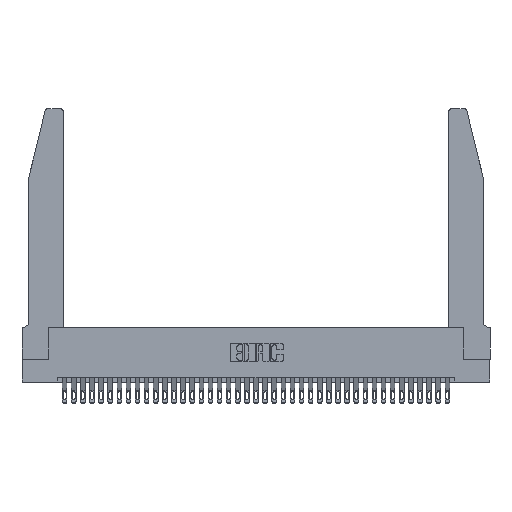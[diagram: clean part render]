
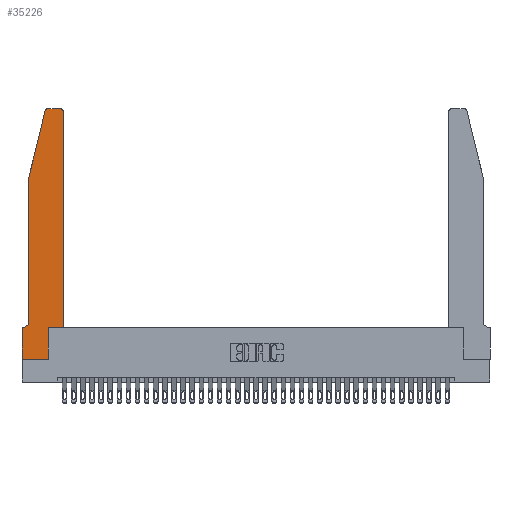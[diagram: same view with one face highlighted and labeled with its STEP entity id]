
A CAD part, top view. The second image highlights one B-rep face of the part: STEP entity #35226.
In plain terms, the highlighted planar face has unit normal (0, 0, 1).
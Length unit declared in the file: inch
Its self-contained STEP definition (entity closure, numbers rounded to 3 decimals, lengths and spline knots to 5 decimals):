
#294 = EDGE_CURVE ( 'NONE', #10274, #26680, #36121, .T. ) ;
#862 = LINE ( 'NONE', #12136, #24023 ) ;
#1189 = LINE ( 'NONE', #4709, #31174 ) ;
#1257 = VERTEX_POINT ( 'NONE', #12791 ) ;
#2645 = EDGE_CURVE ( 'NONE', #26680, #19463, #24543, .T. ) ;
#2766 = ORIENTED_EDGE ( 'NONE', *, *, #25199, .T. ) ;
#3398 = EDGE_CURVE ( 'NONE', #1257, #34797, #37772, .T. ) ;
#3611 = CARTESIAN_POINT ( 'NONE',  ( 0.4505, 0.35, 0.37 ) ) ;
#3882 = DIRECTION ( 'NONE',  ( 0., 1., 0. ) ) ;
#4219 = DIRECTION ( 'NONE',  ( 0., 0., -1. ) ) ;
#4265 = CARTESIAN_POINT ( 'NONE',  ( 0.2865, 0.35, 0.37 ) ) ;
#4335 = AXIS2_PLACEMENT_3D ( 'NONE', #31609, #13985, #34543 ) ;
#4709 = CARTESIAN_POINT ( 'NONE',  ( 0.0755, 0.35, 0.37 ) ) ;
#5029 = CARTESIAN_POINT ( 'NONE',  ( 0.0755, 2., 0.37 ) ) ;
#5697 = ORIENTED_EDGE ( 'NONE', *, *, #32618, .T. ) ;
#7433 = CARTESIAN_POINT ( 'NONE',  ( 0.2865, 0.35, 0.37 ) ) ;
#7866 = ORIENTED_EDGE ( 'NONE', *, *, #37108, .T. ) ;
#8065 = ORIENTED_EDGE ( 'NONE', *, *, #294, .T. ) ;
#8486 = CARTESIAN_POINT ( 'NONE',  ( 0.4505, 0.35, 0.37 ) ) ;
#8924 = CARTESIAN_POINT ( 'NONE',  ( 0., 0., 0.37 ) ) ;
#9117 = DIRECTION ( 'NONE',  ( 0., -1., 0. ) ) ;
#10274 = VERTEX_POINT ( 'NONE', #19923 ) ;
#10420 = VERTEX_POINT ( 'NONE', #20565 ) ;
#10973 = CARTESIAN_POINT ( 'NONE',  ( 0.0055, 0.35, 0.37 ) ) ;
#10982 = PLANE ( 'NONE',  #33431 ) ;
#11278 = CARTESIAN_POINT ( 'NONE',  ( 0.0755, 0.42, 0.37 ) ) ;
#11682 = CARTESIAN_POINT ( 'NONE',  ( 0., 0., 0.37 ) ) ;
#12136 = CARTESIAN_POINT ( 'NONE',  ( 0.2605, 2.75, 0.37 ) ) ;
#12423 = EDGE_CURVE ( 'NONE', #10420, #15939, #29653, .T. ) ;
#12632 = VECTOR ( 'NONE', #32561, 39.37008 ) ;
#12791 = CARTESIAN_POINT ( 'NONE',  ( 0.0755, 2., 0.37 ) ) ;
#13929 = EDGE_CURVE ( 'NONE', #22340, #25320, #33984, .T. ) ;
#13985 = DIRECTION ( 'NONE',  ( 0., 0., 1. ) ) ;
#14031 = ORIENTED_EDGE ( 'NONE', *, *, #27865, .T. ) ;
#14689 = DIRECTION ( 'NONE',  ( 1., 0., 0. ) ) ;
#14968 = EDGE_CURVE ( 'NONE', #27614, #10274, #1189, .T. ) ;
#15150 = CARTESIAN_POINT ( 'NONE',  ( 0.0755, 2., 0.37 ) ) ;
#15884 = ORIENTED_EDGE ( 'NONE', *, *, #28995, .T. ) ;
#15939 = VERTEX_POINT ( 'NONE', #30664 ) ;
#16033 = VECTOR ( 'NONE', #28105, 39.37008 ) ;
#16687 = VECTOR ( 'NONE', #14689, 39.37008 ) ;
#16960 = CARTESIAN_POINT ( 'NONE',  ( 0., 0.35, 0.37 ) ) ;
#17216 = CARTESIAN_POINT ( 'NONE',  ( 0.4205, 2.72, 0.37 ) ) ;
#17730 = ORIENTED_EDGE ( 'NONE', *, *, #30701, .T. ) ;
#18167 = CARTESIAN_POINT ( 'NONE',  ( 0.284, 2.75, 0.37 ) ) ;
#18757 = EDGE_LOOP ( 'NONE', ( #14031, #7866, #15884, #31522, #17730, #23011, #8065, #23949, #2766, #34458, #5697, #21631 ) ) ;
#19463 = VERTEX_POINT ( 'NONE', #32047 ) ;
#19676 = CIRCLE ( 'NONE', #32503, 0.07 ) ;
#19923 = CARTESIAN_POINT ( 'NONE',  ( 0., 0.35, 0.37 ) ) ;
#19924 = DIRECTION ( 'NONE',  ( 1., 0., 0. ) ) ;
#20186 = DIRECTION ( 'NONE',  ( 1., 0., 0. ) ) ;
#20565 = CARTESIAN_POINT ( 'NONE',  ( 0.4505, 2.72, 0.37 ) ) ;
#21631 = ORIENTED_EDGE ( 'NONE', *, *, #12423, .T. ) ;
#22197 = CARTESIAN_POINT ( 'NONE',  ( 0.0055, 0.42, 0.37 ) ) ;
#22340 = VERTEX_POINT ( 'NONE', #7433 ) ;
#22504 = VECTOR ( 'NONE', #3882, 39.37008 ) ;
#22672 = DIRECTION ( 'NONE',  ( -1., 0., 0. ) ) ;
#22796 = CARTESIAN_POINT ( 'NONE',  ( 0.25487, 2.72718, 0.37 ) ) ;
#22971 = DIRECTION ( 'NONE',  ( -0.239, -0.971, 0. ) ) ;
#23011 = ORIENTED_EDGE ( 'NONE', *, *, #14968, .T. ) ;
#23910 = LINE ( 'NONE', #4265, #16033 ) ;
#23949 = ORIENTED_EDGE ( 'NONE', *, *, #2645, .T. ) ;
#24023 = VECTOR ( 'NONE', #29776, 39.37008 ) ;
#24543 = LINE ( 'NONE', #11682, #16687 ) ;
#25151 = DIRECTION ( 'NONE',  ( -1., 0., 0. ) ) ;
#25199 = EDGE_CURVE ( 'NONE', #19463, #22340, #23910, .T. ) ;
#25320 = VERTEX_POINT ( 'NONE', #25691 ) ;
#25691 = CARTESIAN_POINT ( 'NONE',  ( 0.4505, 0.35, 0.37 ) ) ;
#26680 = VERTEX_POINT ( 'NONE', #38084 ) ;
#26759 = VERTEX_POINT ( 'NONE', #18167 ) ;
#27614 = VERTEX_POINT ( 'NONE', #10973 ) ;
#27865 = EDGE_CURVE ( 'NONE', #15939, #26759, #862, .T. ) ;
#28105 = DIRECTION ( 'NONE',  ( 0., 1., 0. ) ) ;
#28995 = EDGE_CURVE ( 'NONE', #32806, #1257, #31248, .T. ) ;
#29653 = CIRCLE ( 'NONE', #35601, 0.03 ) ;
#29776 = DIRECTION ( 'NONE',  ( -1., 0., 0. ) ) ;
#30316 = VECTOR ( 'NONE', #22971, 39.37008 ) ;
#30595 = FACE_OUTER_BOUND ( 'NONE', #18757, .T. ) ;
#30664 = CARTESIAN_POINT ( 'NONE',  ( 0.4205, 2.75, 0.37 ) ) ;
#30701 = EDGE_CURVE ( 'NONE', #34797, #27614, #19676, .T. ) ;
#31174 = VECTOR ( 'NONE', #22672, 39.37008 ) ;
#31220 = LINE ( 'NONE', #3611, #22504 ) ;
#31248 = LINE ( 'NONE', #5029, #30316 ) ;
#31382 = CIRCLE ( 'NONE', #4335, 0.03 ) ;
#31522 = ORIENTED_EDGE ( 'NONE', *, *, #3398, .T. ) ;
#31609 = CARTESIAN_POINT ( 'NONE',  ( 0.284, 2.72, 0.37 ) ) ;
#32047 = CARTESIAN_POINT ( 'NONE',  ( 0.2865, 0., 0.37 ) ) ;
#32503 = AXIS2_PLACEMENT_3D ( 'NONE', #22197, #4219, #25151 ) ;
#32561 = DIRECTION ( 'NONE',  ( 0., -1., 0. ) ) ;
#32618 = EDGE_CURVE ( 'NONE', #25320, #10420, #31220, .T. ) ;
#32806 = VERTEX_POINT ( 'NONE', #22796 ) ;
#33086 = VECTOR ( 'NONE', #38055, 39.37008 ) ;
#33431 = AXIS2_PLACEMENT_3D ( 'NONE', #16960, #37514, #19924 ) ;
#33984 = LINE ( 'NONE', #8486, #33086 ) ;
#34458 = ORIENTED_EDGE ( 'NONE', *, *, #13929, .T. ) ;
#34543 = DIRECTION ( 'NONE',  ( 1., 0., 0. ) ) ;
#34797 = VERTEX_POINT ( 'NONE', #11278 ) ;
#35226 = ADVANCED_FACE ( 'NONE', ( #30595 ), #10982, .T. ) ;
#35601 = AXIS2_PLACEMENT_3D ( 'NONE', #17216, #37766, #20186 ) ;
#36121 = LINE ( 'NONE', #8924, #12632 ) ;
#37108 = EDGE_CURVE ( 'NONE', #26759, #32806, #31382, .T. ) ;
#37514 = DIRECTION ( 'NONE',  ( 0., 0., 1. ) ) ;
#37766 = DIRECTION ( 'NONE',  ( 0., 0., 1. ) ) ;
#37772 = LINE ( 'NONE', #15150, #38701 ) ;
#38055 = DIRECTION ( 'NONE',  ( 1., 0., 0. ) ) ;
#38084 = CARTESIAN_POINT ( 'NONE',  ( 0., 0., 0.37 ) ) ;
#38701 = VECTOR ( 'NONE', #9117, 39.37008 ) ;
